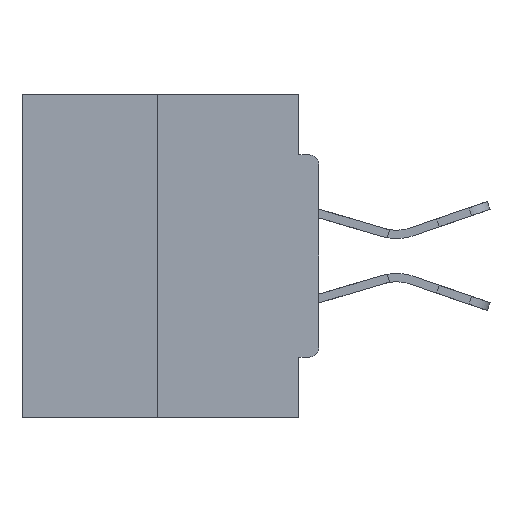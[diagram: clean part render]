
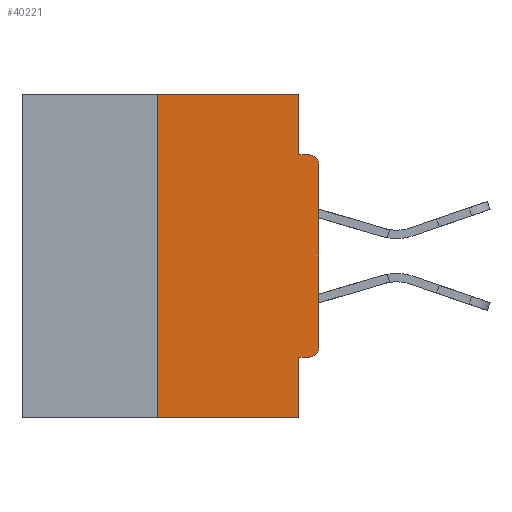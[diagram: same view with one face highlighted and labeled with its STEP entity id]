
A CAD part, left-side view. The second image highlights one B-rep face of the part: STEP entity #40221.
In plain terms, the highlighted planar face has unit normal (-1, 0, 0).
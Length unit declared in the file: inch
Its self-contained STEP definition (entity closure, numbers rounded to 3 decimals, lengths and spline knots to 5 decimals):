
#651 = CARTESIAN_POINT ( 'NONE',  ( 0., 0., 0. ) ) ;
#994 = LINE ( 'NONE', #27997, #35117 ) ;
#1425 = EDGE_CURVE ( 'NONE', #30818, #3852, #8075, .T. ) ;
#1465 = DIRECTION ( 'NONE',  ( 0., 0., -1. ) ) ;
#1918 = DIRECTION ( 'NONE',  ( 0., -1., 0. ) ) ;
#2634 = CARTESIAN_POINT ( 'NONE',  ( 0., 0.031, 0. ) ) ;
#3387 = VECTOR ( 'NONE', #32325, 39.37008 ) ;
#3852 = VERTEX_POINT ( 'NONE', #2634 ) ;
#5582 = CIRCLE ( 'NONE', #9936, 0.015 ) ;
#5600 = EDGE_CURVE ( 'NONE', #42581, #5629, #5582, .T. ) ;
#5629 = VERTEX_POINT ( 'NONE', #15479 ) ;
#6640 = CARTESIAN_POINT ( 'NONE',  ( 0., 0.031, -0.4065 ) ) ;
#6656 = VERTEX_POINT ( 'NONE', #24002 ) ;
#7141 = DIRECTION ( 'NONE',  ( 0., -1., 0. ) ) ;
#7288 = CARTESIAN_POINT ( 'NONE',  ( 0., 0.46, -0.5 ) ) ;
#7335 = DIRECTION ( 'NONE',  ( 0., 0., 1. ) ) ;
#7381 = EDGE_CURVE ( 'NONE', #21571, #6656, #21445, .T. ) ;
#8073 = AXIS2_PLACEMENT_3D ( 'NONE', #8080, #42546, #28981 ) ;
#8075 = LINE ( 'NONE', #11978, #23488 ) ;
#8080 = CARTESIAN_POINT ( 'NONE',  ( 0., 0.015, -0.1085 ) ) ;
#8383 = EDGE_CURVE ( 'NONE', #41736, #14491, #24545, .T. ) ;
#8595 = ORIENTED_EDGE ( 'NONE', *, *, #12974, .F. ) ;
#8832 = FACE_OUTER_BOUND ( 'NONE', #13649, .T. ) ;
#9075 = DIRECTION ( 'NONE',  ( -1., 0., 0. ) ) ;
#9486 = DIRECTION ( 'NONE',  ( 1., 0., 0. ) ) ;
#9770 = AXIS2_PLACEMENT_3D ( 'NONE', #40234, #9486, #12478 ) ;
#9936 = AXIS2_PLACEMENT_3D ( 'NONE', #25659, #9075, #32705 ) ;
#10101 = CARTESIAN_POINT ( 'NONE',  ( 0., 0.015, -0.4065 ) ) ;
#11117 = LINE ( 'NONE', #15455, #28820 ) ;
#11978 = CARTESIAN_POINT ( 'NONE',  ( 0., 0.46, 0. ) ) ;
#12478 = DIRECTION ( 'NONE',  ( 0., 0., -1. ) ) ;
#12974 = EDGE_CURVE ( 'NONE', #3852, #21571, #15021, .T. ) ;
#13649 = EDGE_LOOP ( 'NONE', ( #23894, #28925, #14265, #32210, #24932, #34393, #23180, #21446, #26614, #8595 ) ) ;
#13972 = LINE ( 'NONE', #20293, #41242 ) ;
#14265 = ORIENTED_EDGE ( 'NONE', *, *, #8383, .T. ) ;
#14491 = VERTEX_POINT ( 'NONE', #33487 ) ;
#15021 = LINE ( 'NONE', #42060, #37532 ) ;
#15455 = CARTESIAN_POINT ( 'NONE',  ( 0., 0., -0.4065 ) ) ;
#15479 = CARTESIAN_POINT ( 'NONE',  ( 0., 0., -0.3915 ) ) ;
#16480 = CARTESIAN_POINT ( 'NONE',  ( 0., 0., -0.1085 ) ) ;
#18538 = CARTESIAN_POINT ( 'NONE',  ( 0., 0., -0.0935 ) ) ;
#18801 = CIRCLE ( 'NONE', #8073, 0.015 ) ;
#20007 = EDGE_CURVE ( 'NONE', #32162, #6656, #18801, .T. ) ;
#20293 = CARTESIAN_POINT ( 'NONE',  ( 0., 0.25, 0. ) ) ;
#20763 = CARTESIAN_POINT ( 'NONE',  ( 0., 0.25, -0.5 ) ) ;
#21445 = LINE ( 'NONE', #18538, #3387 ) ;
#21446 = ORIENTED_EDGE ( 'NONE', *, *, #20007, .T. ) ;
#21571 = VERTEX_POINT ( 'NONE', #40351 ) ;
#21887 = DIRECTION ( 'NONE',  ( 0., 1., 0. ) ) ;
#22296 = EDGE_CURVE ( 'NONE', #42581, #23089, #11117, .T. ) ;
#23089 = VERTEX_POINT ( 'NONE', #6640 ) ;
#23180 = ORIENTED_EDGE ( 'NONE', *, *, #43739, .T. ) ;
#23488 = VECTOR ( 'NONE', #1918, 39.37008 ) ;
#23894 = ORIENTED_EDGE ( 'NONE', *, *, #1425, .F. ) ;
#24002 = CARTESIAN_POINT ( 'NONE',  ( 0., 0.015, -0.0935 ) ) ;
#24545 = LINE ( 'NONE', #7288, #40065 ) ;
#24932 = ORIENTED_EDGE ( 'NONE', *, *, #22296, .F. ) ;
#25659 = CARTESIAN_POINT ( 'NONE',  ( 0., 0.015, -0.3915 ) ) ;
#26006 = CARTESIAN_POINT ( 'NONE',  ( 0., 0.25, 0. ) ) ;
#26614 = ORIENTED_EDGE ( 'NONE', *, *, #7381, .F. ) ;
#27823 = VECTOR ( 'NONE', #7335, 39.37008 ) ;
#27997 = CARTESIAN_POINT ( 'NONE',  ( 0., 0.031, -0.5 ) ) ;
#28782 = DIRECTION ( 'NONE',  ( 0., 0., -1. ) ) ;
#28820 = VECTOR ( 'NONE', #21887, 39.37008 ) ;
#28925 = ORIENTED_EDGE ( 'NONE', *, *, #33794, .F. ) ;
#28981 = DIRECTION ( 'NONE',  ( 0., 0., -1. ) ) ;
#29432 = LINE ( 'NONE', #651, #27823 ) ;
#30641 = DIRECTION ( 'NONE',  ( 0., 0., 1. ) ) ;
#30818 = VERTEX_POINT ( 'NONE', #26006 ) ;
#32162 = VERTEX_POINT ( 'NONE', #16480 ) ;
#32210 = ORIENTED_EDGE ( 'NONE', *, *, #39540, .F. ) ;
#32325 = DIRECTION ( 'NONE',  ( 0., -1., 0. ) ) ;
#32705 = DIRECTION ( 'NONE',  ( 0., 0., -1. ) ) ;
#33487 = CARTESIAN_POINT ( 'NONE',  ( 0., 0.031, -0.5 ) ) ;
#33794 = EDGE_CURVE ( 'NONE', #41736, #30818, #13972, .T. ) ;
#34393 = ORIENTED_EDGE ( 'NONE', *, *, #5600, .T. ) ;
#35117 = VECTOR ( 'NONE', #1465, 39.37008 ) ;
#37532 = VECTOR ( 'NONE', #28782, 39.37008 ) ;
#39540 = EDGE_CURVE ( 'NONE', #23089, #14491, #994, .T. ) ;
#40065 = VECTOR ( 'NONE', #7141, 39.37008 ) ;
#40221 = ADVANCED_FACE ( 'NONE', ( #8832 ), #43234, .F. ) ;
#40234 = CARTESIAN_POINT ( 'NONE',  ( 0., 0.46, 0. ) ) ;
#40351 = CARTESIAN_POINT ( 'NONE',  ( 0., 0.031, -0.0935 ) ) ;
#41242 = VECTOR ( 'NONE', #30641, 39.37008 ) ;
#41736 = VERTEX_POINT ( 'NONE', #20763 ) ;
#42060 = CARTESIAN_POINT ( 'NONE',  ( 0., 0.031, 0. ) ) ;
#42546 = DIRECTION ( 'NONE',  ( -1., 0., 0. ) ) ;
#42581 = VERTEX_POINT ( 'NONE', #10101 ) ;
#43234 = PLANE ( 'NONE',  #9770 ) ;
#43739 = EDGE_CURVE ( 'NONE', #5629, #32162, #29432, .T. ) ;
